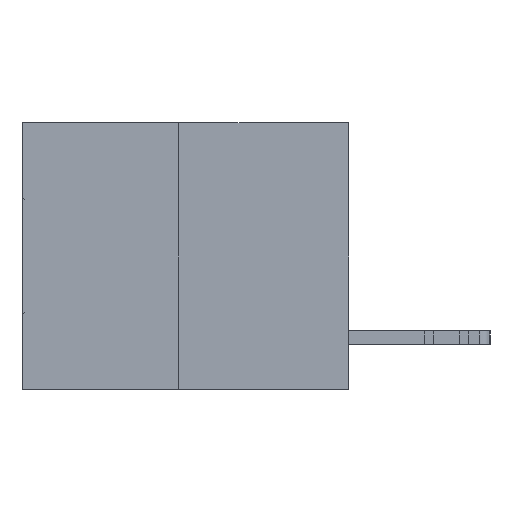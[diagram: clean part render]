
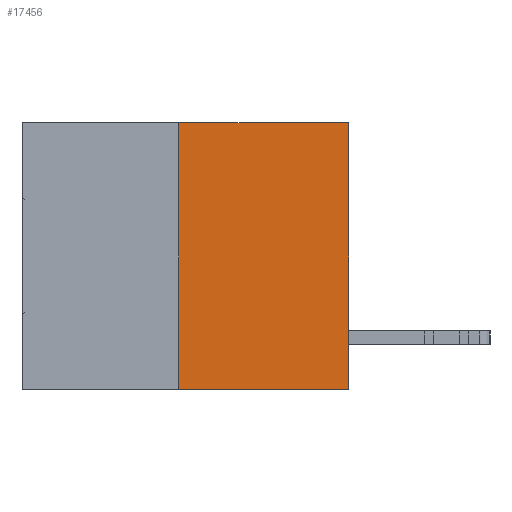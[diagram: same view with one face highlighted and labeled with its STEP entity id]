
A CAD part, left-side view. The second image highlights one B-rep face of the part: STEP entity #17456.
In plain terms, the highlighted planar face has unit normal (-1, 0, 0).
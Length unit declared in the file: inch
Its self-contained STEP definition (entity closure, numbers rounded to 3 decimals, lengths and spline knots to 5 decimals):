
#1824 = CARTESIAN_POINT ( 'NONE',  ( 0., 0.6, 0. ) ) ;
#3506 = VECTOR ( 'NONE', #17019, 39.37008 ) ;
#3758 = VECTOR ( 'NONE', #22295, 39.37008 ) ;
#4105 = DIRECTION ( 'NONE',  ( 0., -1., 0. ) ) ;
#4279 = ORIENTED_EDGE ( 'NONE', *, *, #4973, .T. ) ;
#4513 = CARTESIAN_POINT ( 'NONE',  ( 0., 0.312, -0.49 ) ) ;
#4973 = EDGE_CURVE ( 'NONE', #22829, #10934, #20121, .T. ) ;
#4990 = EDGE_CURVE ( 'NONE', #10934, #25340, #7105, .T. ) ;
#5354 = ORIENTED_EDGE ( 'NONE', *, *, #22362, .F. ) ;
#6190 = CARTESIAN_POINT ( 'NONE',  ( 0., 0., -0.49 ) ) ;
#6411 = FACE_OUTER_BOUND ( 'NONE', #26406, .T. ) ;
#7105 = LINE ( 'NONE', #32593, #3506 ) ;
#8963 = CARTESIAN_POINT ( 'NONE',  ( 0., 0.312, -0.49 ) ) ;
#9379 = CARTESIAN_POINT ( 'NONE',  ( 0., 0.6, -0.49 ) ) ;
#9710 = DIRECTION ( 'NONE',  ( 1., 0., 0. ) ) ;
#10906 = ORIENTED_EDGE ( 'NONE', *, *, #20741, .F. ) ;
#10934 = VERTEX_POINT ( 'NONE', #6190 ) ;
#11824 = LINE ( 'NONE', #14349, #3758 ) ;
#14349 = CARTESIAN_POINT ( 'NONE',  ( 0., 0.6, 0. ) ) ;
#14770 = VECTOR ( 'NONE', #19816, 39.37008 ) ;
#17019 = DIRECTION ( 'NONE',  ( 0., 0., 1. ) ) ;
#17456 = ADVANCED_FACE ( 'NONE', ( #6411 ), #22557, .F. ) ;
#19816 = DIRECTION ( 'NONE',  ( 0., 0., 1. ) ) ;
#20121 = LINE ( 'NONE', #9379, #25771 ) ;
#20741 = EDGE_CURVE ( 'NONE', #22829, #23374, #22513, .T. ) ;
#21330 = CARTESIAN_POINT ( 'NONE',  ( 0., 0., 0. ) ) ;
#22295 = DIRECTION ( 'NONE',  ( 0., -1., 0. ) ) ;
#22362 = EDGE_CURVE ( 'NONE', #23374, #25340, #11824, .T. ) ;
#22513 = LINE ( 'NONE', #4513, #14770 ) ;
#22557 = PLANE ( 'NONE',  #32028 ) ;
#22829 = VERTEX_POINT ( 'NONE', #8963 ) ;
#23374 = VERTEX_POINT ( 'NONE', #25312 ) ;
#25312 = CARTESIAN_POINT ( 'NONE',  ( 0., 0.312, 0. ) ) ;
#25340 = VERTEX_POINT ( 'NONE', #21330 ) ;
#25357 = DIRECTION ( 'NONE',  ( 0., 0., -1. ) ) ;
#25771 = VECTOR ( 'NONE', #4105, 39.37008 ) ;
#26406 = EDGE_LOOP ( 'NONE', ( #10906, #4279, #31584, #5354 ) ) ;
#31584 = ORIENTED_EDGE ( 'NONE', *, *, #4990, .T. ) ;
#32028 = AXIS2_PLACEMENT_3D ( 'NONE', #1824, #9710, #25357 ) ;
#32593 = CARTESIAN_POINT ( 'NONE',  ( 0., 0., 0. ) ) ;
